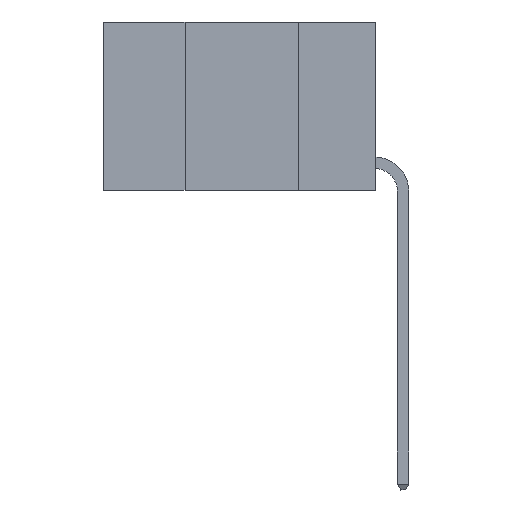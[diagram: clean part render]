
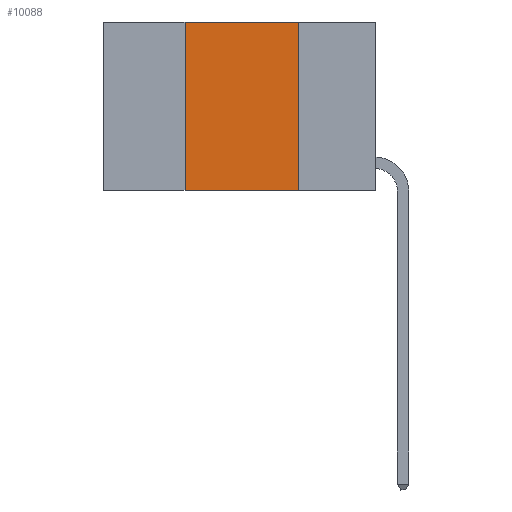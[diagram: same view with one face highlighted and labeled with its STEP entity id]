
A CAD part, left-side view. The second image highlights one B-rep face of the part: STEP entity #10088.
In plain terms, the highlighted planar face has unit normal (-1, 0, 0).
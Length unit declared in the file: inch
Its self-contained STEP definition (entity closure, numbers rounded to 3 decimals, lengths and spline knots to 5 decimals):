
#1584 = ORIENTED_EDGE ( 'NONE', *, *, #16704, .F. ) ;
#1851 = LINE ( 'NONE', #9219, #9595 ) ;
#1883 = DIRECTION ( 'NONE',  ( 0., -1., 0. ) ) ;
#3315 = DIRECTION ( 'NONE',  ( 0., 0., -1. ) ) ;
#5764 = DIRECTION ( 'NONE',  ( 0., 0., 1. ) ) ;
#8625 = CARTESIAN_POINT ( 'NONE',  ( 0., 0.6, 0. ) ) ;
#8907 = VERTEX_POINT ( 'NONE', #22670 ) ;
#9219 = CARTESIAN_POINT ( 'NONE',  ( 0., 0.6, -0.37 ) ) ;
#9595 = VECTOR ( 'NONE', #11411, 39.37008 ) ;
#9927 = DIRECTION ( 'NONE',  ( 1., 0., 0. ) ) ;
#10088 = ADVANCED_FACE ( 'NONE', ( #21484 ), #19445, .F. ) ;
#11411 = DIRECTION ( 'NONE',  ( 0., -1., 0. ) ) ;
#11670 = AXIS2_PLACEMENT_3D ( 'NONE', #28810, #9927, #14603 ) ;
#13726 = CARTESIAN_POINT ( 'NONE',  ( 0., 0.42, 0. ) ) ;
#14240 = VECTOR ( 'NONE', #5764, 39.37008 ) ;
#14603 = DIRECTION ( 'NONE',  ( 0., 0., -1. ) ) ;
#16704 = EDGE_CURVE ( 'NONE', #21669, #8907, #21114, .T. ) ;
#16972 = CARTESIAN_POINT ( 'NONE',  ( 0., 0.42, -0.37 ) ) ;
#19445 = PLANE ( 'NONE',  #11670 ) ;
#19675 = VECTOR ( 'NONE', #3315, 39.37008 ) ;
#20740 = EDGE_LOOP ( 'NONE', ( #26780, #1584, #20917, #23432 ) ) ;
#20917 = ORIENTED_EDGE ( 'NONE', *, *, #30055, .F. ) ;
#21114 = LINE ( 'NONE', #8625, #23343 ) ;
#21484 = FACE_OUTER_BOUND ( 'NONE', #20740, .T. ) ;
#21669 = VERTEX_POINT ( 'NONE', #13726 ) ;
#22401 = CARTESIAN_POINT ( 'NONE',  ( 0., 0.17, 0. ) ) ;
#22670 = CARTESIAN_POINT ( 'NONE',  ( 0., 0.17, 0. ) ) ;
#22789 = CARTESIAN_POINT ( 'NONE',  ( 0., 0.42, 0. ) ) ;
#23343 = VECTOR ( 'NONE', #1883, 39.37008 ) ;
#23432 = ORIENTED_EDGE ( 'NONE', *, *, #24457, .T. ) ;
#24457 = EDGE_CURVE ( 'NONE', #26360, #24866, #1851, .T. ) ;
#24723 = LINE ( 'NONE', #22401, #19675 ) ;
#24866 = VERTEX_POINT ( 'NONE', #30410 ) ;
#26360 = VERTEX_POINT ( 'NONE', #16972 ) ;
#26780 = ORIENTED_EDGE ( 'NONE', *, *, #29217, .F. ) ;
#28810 = CARTESIAN_POINT ( 'NONE',  ( 0., 0.6, 0. ) ) ;
#29217 = EDGE_CURVE ( 'NONE', #8907, #24866, #24723, .T. ) ;
#29498 = LINE ( 'NONE', #22789, #14240 ) ;
#30055 = EDGE_CURVE ( 'NONE', #26360, #21669, #29498, .T. ) ;
#30410 = CARTESIAN_POINT ( 'NONE',  ( 0., 0.17, -0.37 ) ) ;
